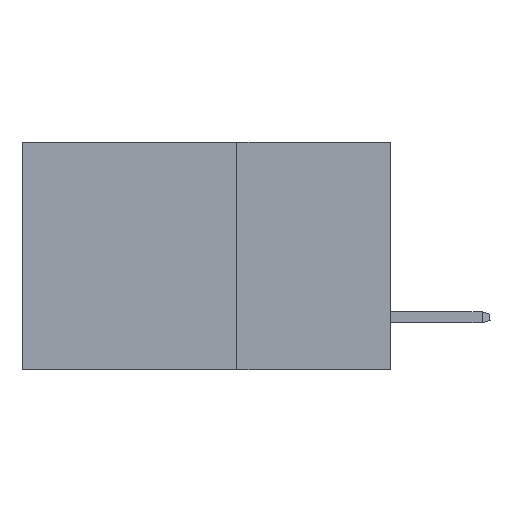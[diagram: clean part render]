
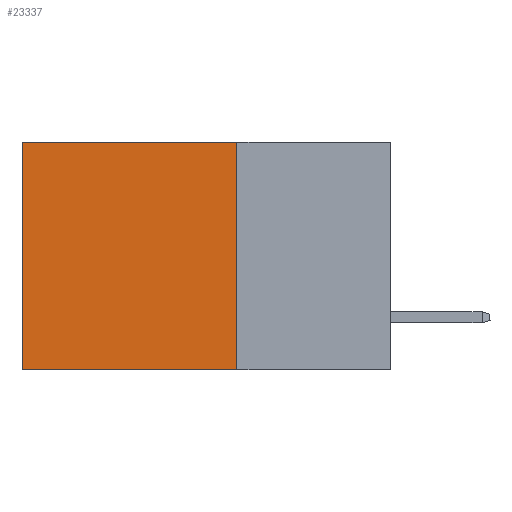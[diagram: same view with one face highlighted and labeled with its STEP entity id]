
A CAD part, left-side view. The second image highlights one B-rep face of the part: STEP entity #23337.
In plain terms, the highlighted planar face has unit normal (-1, 0, 0).
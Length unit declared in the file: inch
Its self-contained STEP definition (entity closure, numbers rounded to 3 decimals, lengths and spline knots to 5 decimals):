
#1347 = LINE ( 'NONE', #12194, #19234 ) ;
#3051 = CARTESIAN_POINT ( 'NONE',  ( 0.2875, 0.6, 0. ) ) ;
#5654 = LINE ( 'NONE', #6185, #32443 ) ;
#6185 = CARTESIAN_POINT ( 'NONE',  ( 0.2875, 0.25, 0. ) ) ;
#6402 = ORIENTED_EDGE ( 'NONE', *, *, #31532, .T. ) ;
#6676 = CARTESIAN_POINT ( 'NONE',  ( 0.2875, 0.6, -0.37 ) ) ;
#7753 = CARTESIAN_POINT ( 'NONE',  ( 0.2875, 0.25, 0. ) ) ;
#8234 = EDGE_LOOP ( 'NONE', ( #6402, #21411, #25604, #31744 ) ) ;
#10382 = DIRECTION ( 'NONE',  ( 0., 0., -1. ) ) ;
#12194 = CARTESIAN_POINT ( 'NONE',  ( 0.2875, 0.25, 0. ) ) ;
#12886 = CARTESIAN_POINT ( 'NONE',  ( 0.2875, 0.25, 0. ) ) ;
#13979 = VERTEX_POINT ( 'NONE', #3051 ) ;
#15132 = EDGE_CURVE ( 'NONE', #26498, #16634, #18636, .T. ) ;
#15399 = PLANE ( 'NONE',  #27118 ) ;
#16350 = LINE ( 'NONE', #21360, #20616 ) ;
#16634 = VERTEX_POINT ( 'NONE', #6676 ) ;
#16690 = DIRECTION ( 'NONE',  ( 0., 0., -1. ) ) ;
#18636 = LINE ( 'NONE', #34324, #35130 ) ;
#19102 = CARTESIAN_POINT ( 'NONE',  ( 0.2875, 0.25, -0.37 ) ) ;
#19234 = VECTOR ( 'NONE', #28953, 39.37008 ) ;
#20616 = VECTOR ( 'NONE', #21890, 39.37008 ) ;
#21360 = CARTESIAN_POINT ( 'NONE',  ( 0.2875, 0.6, 0. ) ) ;
#21411 = ORIENTED_EDGE ( 'NONE', *, *, #15132, .F. ) ;
#21890 = DIRECTION ( 'NONE',  ( 0., 0., -1. ) ) ;
#23337 = ADVANCED_FACE ( 'NONE', ( #29293 ), #15399, .F. ) ;
#25604 = ORIENTED_EDGE ( 'NONE', *, *, #28820, .F. ) ;
#26498 = VERTEX_POINT ( 'NONE', #19102 ) ;
#27118 = AXIS2_PLACEMENT_3D ( 'NONE', #12886, #31971, #10382 ) ;
#28820 = EDGE_CURVE ( 'NONE', #30225, #26498, #5654, .T. ) ;
#28953 = DIRECTION ( 'NONE',  ( 0., 1., 0. ) ) ;
#29293 = FACE_OUTER_BOUND ( 'NONE', #8234, .T. ) ;
#30225 = VERTEX_POINT ( 'NONE', #7753 ) ;
#31532 = EDGE_CURVE ( 'NONE', #13979, #16634, #16350, .T. ) ;
#31659 = DIRECTION ( 'NONE',  ( 0., 1., 0. ) ) ;
#31744 = ORIENTED_EDGE ( 'NONE', *, *, #33534, .T. ) ;
#31971 = DIRECTION ( 'NONE',  ( 1., 0., 0. ) ) ;
#32443 = VECTOR ( 'NONE', #16690, 39.37008 ) ;
#33534 = EDGE_CURVE ( 'NONE', #30225, #13979, #1347, .T. ) ;
#34324 = CARTESIAN_POINT ( 'NONE',  ( 0.2875, 0.25, -0.37 ) ) ;
#35130 = VECTOR ( 'NONE', #31659, 39.37008 ) ;
